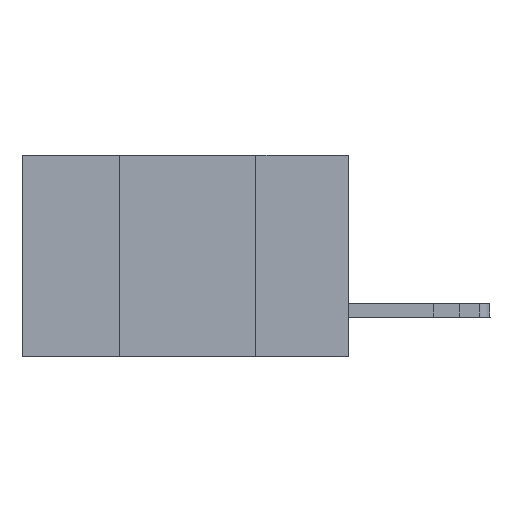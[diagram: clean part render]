
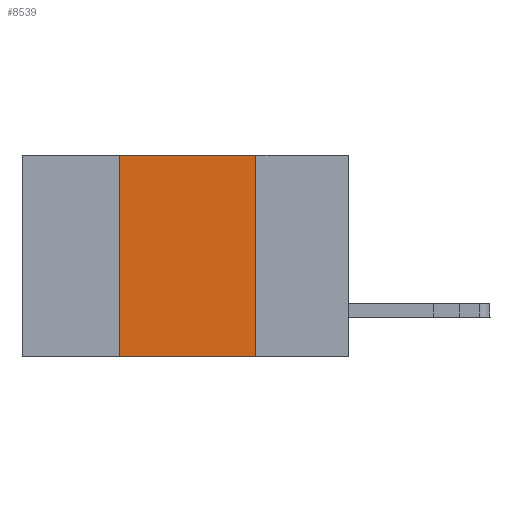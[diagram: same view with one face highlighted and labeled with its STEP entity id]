
A CAD part, left-side view. The second image highlights one B-rep face of the part: STEP entity #8539.
In plain terms, the highlighted planar face has unit normal (-1, 0, 0).
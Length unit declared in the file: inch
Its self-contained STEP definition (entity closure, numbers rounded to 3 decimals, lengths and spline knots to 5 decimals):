
#348 = PLANE ( 'NONE',  #16358 ) ;
#1556 = ORIENTED_EDGE ( 'NONE', *, *, #5525, .F. ) ;
#3115 = LINE ( 'NONE', #8837, #5155 ) ;
#3239 = DIRECTION ( 'NONE',  ( 0., -1., 0. ) ) ;
#3273 = CARTESIAN_POINT ( 'NONE',  ( 0., 0.42, 0. ) ) ;
#3916 = FACE_OUTER_BOUND ( 'NONE', #9692, .T. ) ;
#3976 = EDGE_CURVE ( 'NONE', #15405, #18575, #4933, .T. ) ;
#4044 = DIRECTION ( 'NONE',  ( 1., 0., 0. ) ) ;
#4684 = VERTEX_POINT ( 'NONE', #23772 ) ;
#4933 = LINE ( 'NONE', #3273, #23263 ) ;
#5155 = VECTOR ( 'NONE', #3239, 39.37008 ) ;
#5525 = EDGE_CURVE ( 'NONE', #18575, #11226, #24470, .T. ) ;
#7511 = VECTOR ( 'NONE', #11785, 39.37008 ) ;
#8539 = ADVANCED_FACE ( 'NONE', ( #3916 ), #348, .F. ) ;
#8837 = CARTESIAN_POINT ( 'NONE',  ( 0., 0.6, -0.37 ) ) ;
#9097 = CARTESIAN_POINT ( 'NONE',  ( 0., 0.17, 0. ) ) ;
#9692 = EDGE_LOOP ( 'NONE', ( #11738, #1556, #17432, #13294 ) ) ;
#9898 = CARTESIAN_POINT ( 'NONE',  ( 0., 0.6, 0. ) ) ;
#10882 = DIRECTION ( 'NONE',  ( 0., -1., 0. ) ) ;
#10991 = EDGE_CURVE ( 'NONE', #11226, #4684, #17395, .T. ) ;
#11226 = VERTEX_POINT ( 'NONE', #9097 ) ;
#11623 = CARTESIAN_POINT ( 'NONE',  ( 0., 0.42, -0.37 ) ) ;
#11738 = ORIENTED_EDGE ( 'NONE', *, *, #10991, .F. ) ;
#11785 = DIRECTION ( 'NONE',  ( 0., 0., -1. ) ) ;
#12686 = DIRECTION ( 'NONE',  ( 0., 0., 1. ) ) ;
#13198 = CARTESIAN_POINT ( 'NONE',  ( 0., 0.17, 0. ) ) ;
#13294 = ORIENTED_EDGE ( 'NONE', *, *, #23727, .T. ) ;
#13840 = VECTOR ( 'NONE', #10882, 39.37008 ) ;
#14109 = CARTESIAN_POINT ( 'NONE',  ( 0., 0.42, 0. ) ) ;
#15405 = VERTEX_POINT ( 'NONE', #11623 ) ;
#16358 = AXIS2_PLACEMENT_3D ( 'NONE', #9898, #4044, #21318 ) ;
#17395 = LINE ( 'NONE', #13198, #7511 ) ;
#17432 = ORIENTED_EDGE ( 'NONE', *, *, #3976, .F. ) ;
#18575 = VERTEX_POINT ( 'NONE', #14109 ) ;
#21318 = DIRECTION ( 'NONE',  ( 0., 0., -1. ) ) ;
#22565 = CARTESIAN_POINT ( 'NONE',  ( 0., 0.6, 0. ) ) ;
#23263 = VECTOR ( 'NONE', #12686, 39.37008 ) ;
#23727 = EDGE_CURVE ( 'NONE', #15405, #4684, #3115, .T. ) ;
#23772 = CARTESIAN_POINT ( 'NONE',  ( 0., 0.17, -0.37 ) ) ;
#24470 = LINE ( 'NONE', #22565, #13840 ) ;
